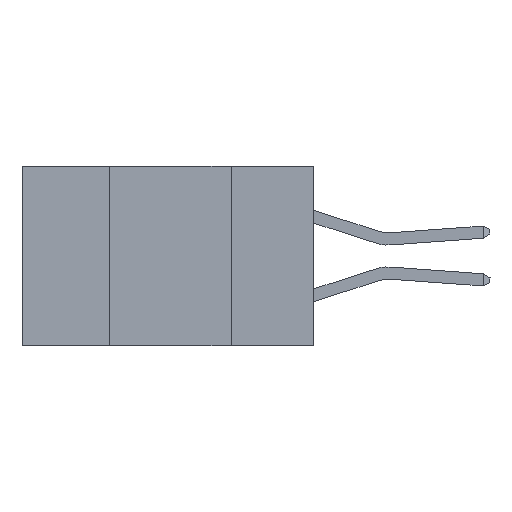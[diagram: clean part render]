
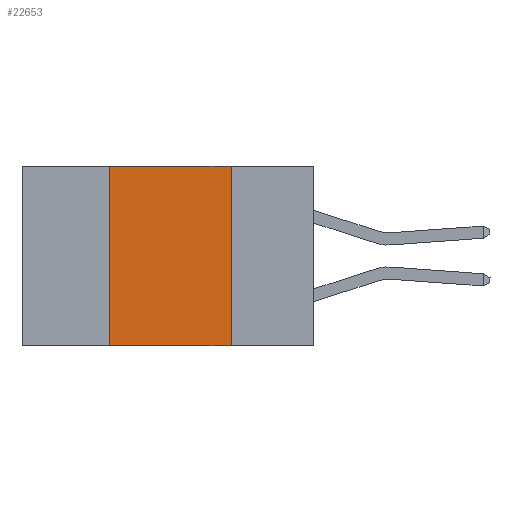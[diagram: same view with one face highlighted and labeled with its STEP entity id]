
A CAD part, left-side view. The second image highlights one B-rep face of the part: STEP entity #22653.
In plain terms, the highlighted planar face has unit normal (-1, 0, 0).
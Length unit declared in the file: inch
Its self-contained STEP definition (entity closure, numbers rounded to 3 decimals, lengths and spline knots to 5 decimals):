
#743 = DIRECTION ( 'NONE',  ( 0., 0., 1. ) ) ;
#3332 = DIRECTION ( 'NONE',  ( 0., 0., -1. ) ) ;
#4465 = EDGE_CURVE ( 'NONE', #14619, #4584, #24357, .T. ) ;
#4584 = VERTEX_POINT ( 'NONE', #12015 ) ;
#4960 = DIRECTION ( 'NONE',  ( 0., -1., 0. ) ) ;
#5819 = EDGE_CURVE ( 'NONE', #19765, #21131, #24238, .T. ) ;
#6581 = EDGE_CURVE ( 'NONE', #21131, #4584, #39772, .T. ) ;
#6885 = AXIS2_PLACEMENT_3D ( 'NONE', #10342, #13557, #26641 ) ;
#10342 = CARTESIAN_POINT ( 'NONE',  ( 0., 0.6, 0. ) ) ;
#12015 = CARTESIAN_POINT ( 'NONE',  ( 0., 0.17, -0.37 ) ) ;
#12567 = CARTESIAN_POINT ( 'NONE',  ( 0., 0.42, -0.37 ) ) ;
#13557 = DIRECTION ( 'NONE',  ( 1., 0., 0. ) ) ;
#14578 = CARTESIAN_POINT ( 'NONE',  ( 0., 0.17, 0. ) ) ;
#14619 = VERTEX_POINT ( 'NONE', #12567 ) ;
#18245 = FACE_OUTER_BOUND ( 'NONE', #26314, .T. ) ;
#19683 = ORIENTED_EDGE ( 'NONE', *, *, #4465, .T. ) ;
#19765 = VERTEX_POINT ( 'NONE', #32533 ) ;
#20574 = CARTESIAN_POINT ( 'NONE',  ( 0., 0.42, 0. ) ) ;
#20662 = ORIENTED_EDGE ( 'NONE', *, *, #5819, .F. ) ;
#20687 = VECTOR ( 'NONE', #33431, 39.37008 ) ;
#21131 = VERTEX_POINT ( 'NONE', #14578 ) ;
#21668 = VECTOR ( 'NONE', #3332, 39.37008 ) ;
#22653 = ADVANCED_FACE ( 'NONE', ( #18245 ), #26783, .F. ) ;
#24238 = LINE ( 'NONE', #30612, #20687 ) ;
#24357 = LINE ( 'NONE', #30854, #24845 ) ;
#24845 = VECTOR ( 'NONE', #4960, 39.37008 ) ;
#25985 = LINE ( 'NONE', #20574, #34060 ) ;
#26314 = EDGE_LOOP ( 'NONE', ( #39192, #20662, #32075, #19683 ) ) ;
#26641 = DIRECTION ( 'NONE',  ( 0., 0., -1. ) ) ;
#26783 = PLANE ( 'NONE',  #6885 ) ;
#30612 = CARTESIAN_POINT ( 'NONE',  ( 0., 0.6, 0. ) ) ;
#30854 = CARTESIAN_POINT ( 'NONE',  ( 0., 0.6, -0.37 ) ) ;
#32075 = ORIENTED_EDGE ( 'NONE', *, *, #38224, .F. ) ;
#32533 = CARTESIAN_POINT ( 'NONE',  ( 0., 0.42, 0. ) ) ;
#33431 = DIRECTION ( 'NONE',  ( 0., -1., 0. ) ) ;
#34060 = VECTOR ( 'NONE', #743, 39.37008 ) ;
#35427 = CARTESIAN_POINT ( 'NONE',  ( 0., 0.17, 0. ) ) ;
#38224 = EDGE_CURVE ( 'NONE', #14619, #19765, #25985, .T. ) ;
#39192 = ORIENTED_EDGE ( 'NONE', *, *, #6581, .F. ) ;
#39772 = LINE ( 'NONE', #35427, #21668 ) ;
